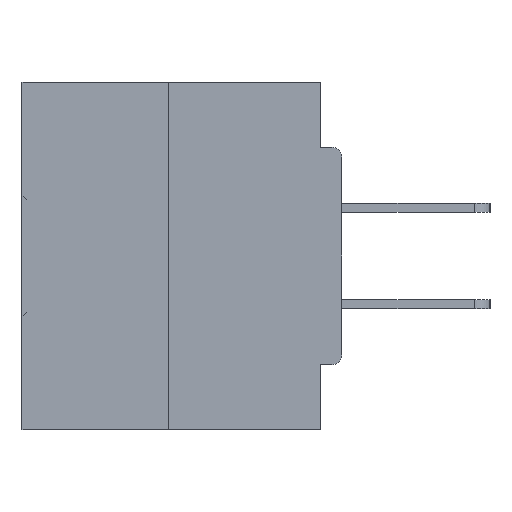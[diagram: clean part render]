
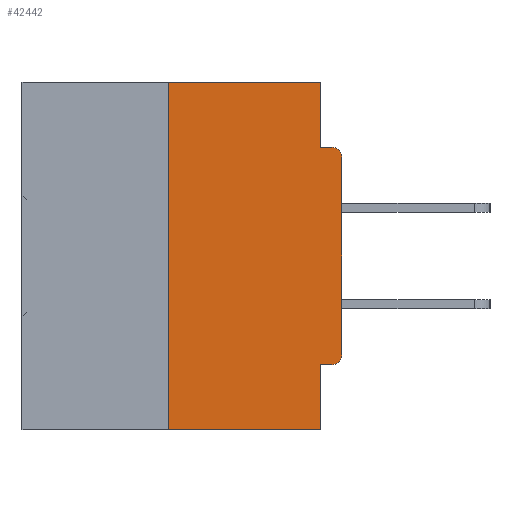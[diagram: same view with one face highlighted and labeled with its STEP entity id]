
A CAD part, left-side view. The second image highlights one B-rep face of the part: STEP entity #42442.
In plain terms, the highlighted planar face has unit normal (-1, 0, 0).
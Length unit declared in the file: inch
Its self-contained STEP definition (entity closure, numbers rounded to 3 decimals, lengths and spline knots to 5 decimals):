
#159 = LINE ( 'NONE', #29606, #15563 ) ;
#895 = VECTOR ( 'NONE', #23763, 39.37008 ) ;
#1092 = CARTESIAN_POINT ( 'NONE',  ( 0., 0.015, -0.3915 ) ) ;
#1211 = VECTOR ( 'NONE', #24953, 39.37008 ) ;
#5345 = DIRECTION ( 'NONE',  ( 0., 0., -1. ) ) ;
#5662 = ORIENTED_EDGE ( 'NONE', *, *, #17311, .F. ) ;
#5772 = LINE ( 'NONE', #33650, #10163 ) ;
#6995 = VERTEX_POINT ( 'NONE', #17416 ) ;
#7856 = CARTESIAN_POINT ( 'NONE',  ( 0., 0.015, -0.1085 ) ) ;
#8055 = CARTESIAN_POINT ( 'NONE',  ( 0., 0.25, -0.5 ) ) ;
#8392 = EDGE_CURVE ( 'NONE', #35950, #29388, #28316, .T. ) ;
#9485 = CARTESIAN_POINT ( 'NONE',  ( 0., 0., -0.0935 ) ) ;
#9730 = VERTEX_POINT ( 'NONE', #36398 ) ;
#10163 = VECTOR ( 'NONE', #5345, 39.37008 ) ;
#10340 = ORIENTED_EDGE ( 'NONE', *, *, #22956, .T. ) ;
#10467 = CARTESIAN_POINT ( 'NONE',  ( 0., 0.015, -0.0935 ) ) ;
#10554 = ORIENTED_EDGE ( 'NONE', *, *, #30625, .T. ) ;
#10663 = DIRECTION ( 'NONE',  ( 0., 1., 0. ) ) ;
#12428 = VERTEX_POINT ( 'NONE', #22820 ) ;
#12667 = DIRECTION ( 'NONE',  ( 1., 0., 0. ) ) ;
#12815 = DIRECTION ( 'NONE',  ( 0., -1., 0. ) ) ;
#13029 = CIRCLE ( 'NONE', #42948, 0.015 ) ;
#13067 = VERTEX_POINT ( 'NONE', #18167 ) ;
#13909 = DIRECTION ( 'NONE',  ( 0., -1., 0. ) ) ;
#14385 = VERTEX_POINT ( 'NONE', #37017 ) ;
#14709 = VERTEX_POINT ( 'NONE', #19377 ) ;
#15563 = VECTOR ( 'NONE', #32868, 39.37008 ) ;
#15934 = CARTESIAN_POINT ( 'NONE',  ( 0., 0.46, -0.5 ) ) ;
#15986 = ORIENTED_EDGE ( 'NONE', *, *, #36466, .T. ) ;
#16263 = VERTEX_POINT ( 'NONE', #10467 ) ;
#16809 = ORIENTED_EDGE ( 'NONE', *, *, #20317, .F. ) ;
#17311 = EDGE_CURVE ( 'NONE', #13067, #29388, #23169, .T. ) ;
#17416 = CARTESIAN_POINT ( 'NONE',  ( 0., 0., -0.1085 ) ) ;
#18167 = CARTESIAN_POINT ( 'NONE',  ( 0., 0.031, -0.4065 ) ) ;
#18835 = ORIENTED_EDGE ( 'NONE', *, *, #30610, .F. ) ;
#19377 = CARTESIAN_POINT ( 'NONE',  ( 0., 0.015, -0.4065 ) ) ;
#20317 = EDGE_CURVE ( 'NONE', #44850, #16263, #31155, .T. ) ;
#21444 = EDGE_CURVE ( 'NONE', #9730, #14385, #31668, .T. ) ;
#22627 = FACE_OUTER_BOUND ( 'NONE', #28548, .T. ) ;
#22820 = CARTESIAN_POINT ( 'NONE',  ( 0., 0., -0.3915 ) ) ;
#22956 = EDGE_CURVE ( 'NONE', #14709, #12428, #38662, .T. ) ;
#23169 = LINE ( 'NONE', #42361, #1211 ) ;
#23237 = PLANE ( 'NONE',  #30421 ) ;
#23763 = DIRECTION ( 'NONE',  ( 0., -1., 0. ) ) ;
#23931 = CARTESIAN_POINT ( 'NONE',  ( 0., 0.031, -0.5 ) ) ;
#24953 = DIRECTION ( 'NONE',  ( 0., 0., -1. ) ) ;
#25102 = ORIENTED_EDGE ( 'NONE', *, *, #39952, .F. ) ;
#26169 = DIRECTION ( 'NONE',  ( 0., 0., 1. ) ) ;
#26622 = CARTESIAN_POINT ( 'NONE',  ( 0., 0.46, 0. ) ) ;
#28060 = LINE ( 'NONE', #35440, #36910 ) ;
#28316 = LINE ( 'NONE', #15934, #34938 ) ;
#28548 = EDGE_LOOP ( 'NONE', ( #31539, #18835, #33899, #5662, #25102, #10340, #10554, #15986, #16809, #40006 ) ) ;
#28575 = DIRECTION ( 'NONE',  ( -1., 0., 0. ) ) ;
#29313 = CARTESIAN_POINT ( 'NONE',  ( 0., 0.46, 0. ) ) ;
#29388 = VERTEX_POINT ( 'NONE', #23931 ) ;
#29403 = CARTESIAN_POINT ( 'NONE',  ( 0., 0.031, -0.0935 ) ) ;
#29606 = CARTESIAN_POINT ( 'NONE',  ( 0., 0.25, 0. ) ) ;
#29695 = EDGE_CURVE ( 'NONE', #14385, #44850, #5772, .T. ) ;
#30421 = AXIS2_PLACEMENT_3D ( 'NONE', #26622, #12667, #40969 ) ;
#30610 = EDGE_CURVE ( 'NONE', #35950, #9730, #159, .T. ) ;
#30625 = EDGE_CURVE ( 'NONE', #12428, #6995, #43125, .T. ) ;
#31155 = LINE ( 'NONE', #9485, #895 ) ;
#31539 = ORIENTED_EDGE ( 'NONE', *, *, #21444, .F. ) ;
#31668 = LINE ( 'NONE', #29313, #38803 ) ;
#32029 = DIRECTION ( 'NONE',  ( -1., 0., 0. ) ) ;
#32868 = DIRECTION ( 'NONE',  ( 0., 0., 1. ) ) ;
#33650 = CARTESIAN_POINT ( 'NONE',  ( 0., 0.031, 0. ) ) ;
#33899 = ORIENTED_EDGE ( 'NONE', *, *, #8392, .T. ) ;
#34938 = VECTOR ( 'NONE', #13909, 39.37008 ) ;
#35440 = CARTESIAN_POINT ( 'NONE',  ( 0., 0., -0.4065 ) ) ;
#35696 = DIRECTION ( 'NONE',  ( 0., 0., -1. ) ) ;
#35950 = VERTEX_POINT ( 'NONE', #8055 ) ;
#36174 = DIRECTION ( 'NONE',  ( 0., 0., -1. ) ) ;
#36398 = CARTESIAN_POINT ( 'NONE',  ( 0., 0.25, 0. ) ) ;
#36466 = EDGE_CURVE ( 'NONE', #6995, #16263, #13029, .T. ) ;
#36910 = VECTOR ( 'NONE', #10663, 39.37008 ) ;
#37017 = CARTESIAN_POINT ( 'NONE',  ( 0., 0.031, 0. ) ) ;
#38074 = AXIS2_PLACEMENT_3D ( 'NONE', #1092, #32029, #36174 ) ;
#38662 = CIRCLE ( 'NONE', #38074, 0.015 ) ;
#38803 = VECTOR ( 'NONE', #12815, 39.37008 ) ;
#39952 = EDGE_CURVE ( 'NONE', #14709, #13067, #28060, .T. ) ;
#40006 = ORIENTED_EDGE ( 'NONE', *, *, #29695, .F. ) ;
#40969 = DIRECTION ( 'NONE',  ( 0., 0., -1. ) ) ;
#42007 = VECTOR ( 'NONE', #26169, 39.37008 ) ;
#42361 = CARTESIAN_POINT ( 'NONE',  ( 0., 0.031, -0.5 ) ) ;
#42442 = ADVANCED_FACE ( 'NONE', ( #22627 ), #23237, .F. ) ;
#42948 = AXIS2_PLACEMENT_3D ( 'NONE', #7856, #28575, #35696 ) ;
#43125 = LINE ( 'NONE', #43454, #42007 ) ;
#43454 = CARTESIAN_POINT ( 'NONE',  ( 0., 0., 0. ) ) ;
#44850 = VERTEX_POINT ( 'NONE', #29403 ) ;
